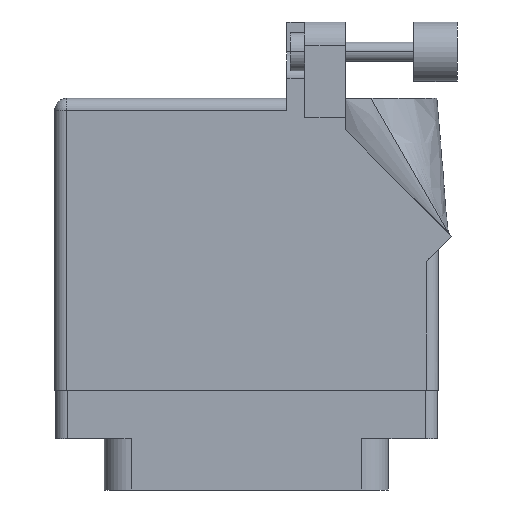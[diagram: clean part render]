
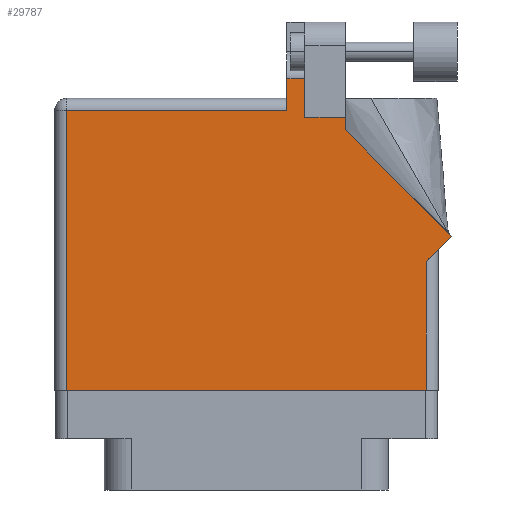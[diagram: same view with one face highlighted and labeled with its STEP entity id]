
A CAD part, front view. The second image highlights one B-rep face of the part: STEP entity #29787.
In plain terms, the highlighted face is planar.
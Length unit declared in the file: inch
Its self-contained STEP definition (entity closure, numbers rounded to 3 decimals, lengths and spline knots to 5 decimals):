
#195 = CARTESIAN_POINT ( 'NONE',  ( 0.212, 1.5315, 0.455 ) ) ;
#367 = VERTEX_POINT ( 'NONE', #30083 ) ;
#734 = CARTESIAN_POINT ( 'NONE',  ( 0.212, 1.43, 0.455 ) ) ;
#936 = ORIENTED_EDGE ( 'NONE', *, *, #5712, .T. ) ;
#1004 = DIRECTION ( 'NONE',  ( 1., 0., 0. ) ) ;
#1104 = EDGE_CURVE ( 'NONE', #22851, #10649, #34931, .T. ) ;
#1128 = VERTEX_POINT ( 'NONE', #195 ) ;
#1630 = ORIENTED_EDGE ( 'NONE', *, *, #6577, .T. ) ;
#1917 = ORIENTED_EDGE ( 'NONE', *, *, #10095, .T. ) ;
#2297 = CARTESIAN_POINT ( 'NONE',  ( 0.63677, 1.5315, 0.455 ) ) ;
#2731 = CARTESIAN_POINT ( 'NONE',  ( 0.519, 1.33, 0.455 ) ) ;
#3811 = DIRECTION ( 'NONE',  ( 0., 1., 0. ) ) ;
#3818 = VERTEX_POINT ( 'NONE', #22883 ) ;
#3819 = ORIENTED_EDGE ( 'NONE', *, *, #1104, .T. ) ;
#4315 = VECTOR ( 'NONE', #26363, 39.37008 ) ;
#5154 = DIRECTION ( 'NONE',  ( -1., 0., 0. ) ) ;
#5489 = ORIENTED_EDGE ( 'NONE', *, *, #18725, .T. ) ;
#5712 = EDGE_CURVE ( 'NONE', #1128, #3818, #7416, .T. ) ;
#5739 = LINE ( 'NONE', #6538, #9821 ) ;
#6226 = LINE ( 'NONE', #2297, #10563 ) ;
#6538 = CARTESIAN_POINT ( 'NONE',  ( 0.519, 1.26442, 0.455 ) ) ;
#6577 = EDGE_CURVE ( 'NONE', #9343, #34367, #24400, .T. ) ;
#6728 = CARTESIAN_POINT ( 'NONE',  ( 0.306, 1.33, 0.455 ) ) ;
#6744 = LINE ( 'NONE', #11952, #29100 ) ;
#7402 = CARTESIAN_POINT ( 'NONE',  ( -1.005, 1.368, 0.455 ) ) ;
#7416 = LINE ( 'NONE', #734, #20495 ) ;
#7683 = FACE_OUTER_BOUND ( 'NONE', #7882, .T. ) ;
#7882 = EDGE_LOOP ( 'NONE', ( #3819, #12353, #936, #5489, #19819, #7983, #33679, #22103, #1630, #21412, #1917 ) ) ;
#7983 = ORIENTED_EDGE ( 'NONE', *, *, #13610, .T. ) ;
#8113 = CARTESIAN_POINT ( 'NONE',  ( -0.943, 1.368, 0.455 ) ) ;
#9306 = DIRECTION ( 'NONE',  ( 0., -1., 0. ) ) ;
#9343 = VERTEX_POINT ( 'NONE', #30985 ) ;
#9461 = VECTOR ( 'NONE', #14478, 39.37008 ) ;
#9550 = LINE ( 'NONE', #7402, #24018 ) ;
#9821 = VECTOR ( 'NONE', #29325, 39.37008 ) ;
#10095 = EDGE_CURVE ( 'NONE', #27200, #22851, #25500, .T. ) ;
#10563 = VECTOR ( 'NONE', #5154, 39.37008 ) ;
#10649 = VERTEX_POINT ( 'NONE', #23760 ) ;
#11128 = AXIS2_PLACEMENT_3D ( 'NONE', #32206, #12496, #20962 ) ;
#11952 = CARTESIAN_POINT ( 'NONE',  ( 0.943, 0.637, 0.455 ) ) ;
#12353 = ORIENTED_EDGE ( 'NONE', *, *, #32385, .T. ) ;
#12496 = DIRECTION ( 'NONE',  ( 0., 0., -1. ) ) ;
#13368 = VERTEX_POINT ( 'NONE', #30127 ) ;
#13610 = EDGE_CURVE ( 'NONE', #32408, #367, #14712, .T. ) ;
#13620 = VECTOR ( 'NONE', #28874, 39.37008 ) ;
#14478 = DIRECTION ( 'NONE',  ( 0., 1., 0. ) ) ;
#14712 = LINE ( 'NONE', #31460, #23507 ) ;
#16170 = CARTESIAN_POINT ( 'NONE',  ( 1.07571, 0.70771, 0.455 ) ) ;
#17589 = DIRECTION ( 'NONE',  ( 0.707, 0.707, 0. ) ) ;
#18725 = EDGE_CURVE ( 'NONE', #3818, #22668, #9550, .T. ) ;
#19053 = EDGE_CURVE ( 'NONE', #22668, #32408, #31530, .T. ) ;
#19819 = ORIENTED_EDGE ( 'NONE', *, *, #19053, .T. ) ;
#20023 = CARTESIAN_POINT ( 'NONE',  ( 1.005, 0.637, 0.455 ) ) ;
#20495 = VECTOR ( 'NONE', #9306, 39.37008 ) ;
#20836 = PLANE ( 'NONE',  #11128 ) ;
#20962 = DIRECTION ( 'NONE',  ( -1., 0., 0. ) ) ;
#21412 = ORIENTED_EDGE ( 'NONE', *, *, #28734, .T. ) ;
#21705 = DIRECTION ( 'NONE',  ( -0.707, 0.707, 0. ) ) ;
#22103 = ORIENTED_EDGE ( 'NONE', *, *, #34010, .T. ) ;
#22312 = EDGE_CURVE ( 'NONE', #367, #13368, #6744, .T. ) ;
#22668 = VERTEX_POINT ( 'NONE', #8113 ) ;
#22851 = VERTEX_POINT ( 'NONE', #6728 ) ;
#22883 = CARTESIAN_POINT ( 'NONE',  ( 0.212, 1.368, 0.455 ) ) ;
#23507 = VECTOR ( 'NONE', #1004, 39.37008 ) ;
#23628 = CARTESIAN_POINT ( 'NONE',  ( -0.943, -0.1, 0.455 ) ) ;
#23760 = CARTESIAN_POINT ( 'NONE',  ( 0.306, 1.5315, 0.455 ) ) ;
#24018 = VECTOR ( 'NONE', #32546, 39.37008 ) ;
#24400 = LINE ( 'NONE', #16170, #25740 ) ;
#25500 = LINE ( 'NONE', #26658, #13620 ) ;
#25575 = CARTESIAN_POINT ( 'NONE',  ( 0.306, 1.33, 0.455 ) ) ;
#25740 = VECTOR ( 'NONE', #21705, 39.37008 ) ;
#26363 = DIRECTION ( 'NONE',  ( 0., -1., 0. ) ) ;
#26658 = CARTESIAN_POINT ( 'NONE',  ( 0.519, 1.33, 0.455 ) ) ;
#27191 = CARTESIAN_POINT ( 'NONE',  ( -0.943, -0.1, 0.455 ) ) ;
#27200 = VERTEX_POINT ( 'NONE', #2731 ) ;
#28734 = EDGE_CURVE ( 'NONE', #34367, #27200, #5739, .T. ) ;
#28874 = DIRECTION ( 'NONE',  ( -1., 0., 0. ) ) ;
#29100 = VECTOR ( 'NONE', #3811, 39.37008 ) ;
#29323 = VECTOR ( 'NONE', #17589, 39.37008 ) ;
#29325 = DIRECTION ( 'NONE',  ( 0., 1., 0. ) ) ;
#29787 = ADVANCED_FACE ( 'NONE', ( #7683 ), #20836, .F. ) ;
#30083 = CARTESIAN_POINT ( 'NONE',  ( 0.943, -0.1, 0.455 ) ) ;
#30127 = CARTESIAN_POINT ( 'NONE',  ( 0.943, 0.575, 0.455 ) ) ;
#30644 = CARTESIAN_POINT ( 'NONE',  ( 0.519, 1.26442, 0.455 ) ) ;
#30985 = CARTESIAN_POINT ( 'NONE',  ( 1.07571, 0.70771, 0.455 ) ) ;
#31115 = LINE ( 'NONE', #20023, #29323 ) ;
#31460 = CARTESIAN_POINT ( 'NONE',  ( -1.005, -0.1, 0.455 ) ) ;
#31530 = LINE ( 'NONE', #23628, #4315 ) ;
#32206 = CARTESIAN_POINT ( 'NONE',  ( -1.005, 1.43, 0.455 ) ) ;
#32385 = EDGE_CURVE ( 'NONE', #10649, #1128, #6226, .T. ) ;
#32408 = VERTEX_POINT ( 'NONE', #27191 ) ;
#32546 = DIRECTION ( 'NONE',  ( -1., 0., 0. ) ) ;
#33679 = ORIENTED_EDGE ( 'NONE', *, *, #22312, .T. ) ;
#34010 = EDGE_CURVE ( 'NONE', #13368, #9343, #31115, .T. ) ;
#34367 = VERTEX_POINT ( 'NONE', #30644 ) ;
#34931 = LINE ( 'NONE', #25575, #9461 ) ;
